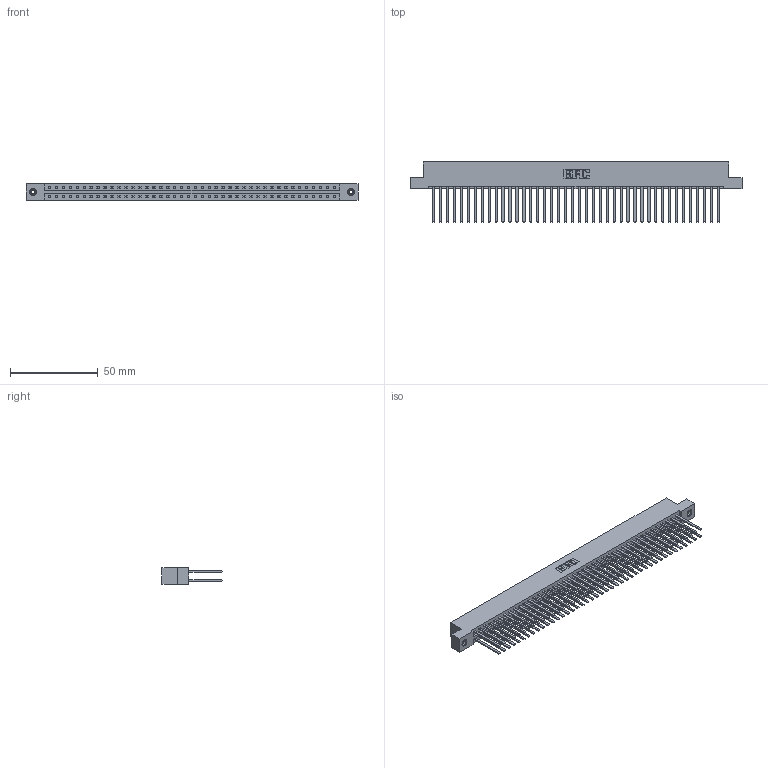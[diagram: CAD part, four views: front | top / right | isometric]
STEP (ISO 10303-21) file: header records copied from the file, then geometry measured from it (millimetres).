
FILE_DESCRIPTION (( 'STEP AP203' ), '1' );
FILE_NAME ('387-084-544-208.STEP', '2018-09-23T22:19:50', ( '' ), ( '' ), 'SwSTEP 2.0', 'SolidWorks 2016', '' );
FILE_SCHEMA (( 'CONFIG_CONTROL_DESIGN' ));
Length unit declared in the file: inch
Products named in the file (4): 337 Part_Flush Mounting Lugs - 0.156 Dia-TI; 345-292-001_345-293-144; 345-250-001_345-250-003-102; 387-084-544-208
Assembly tree (87 placements, depth 2):
  387-084-544-208
    337 Part_Flush Mounting Lugs - 0.156 Dia-TI
    345-292-001_345-293-144  x84
    345-250-001_345-250-003-102  x2
Bounding box: 189.43 x 34.3 x 9.4 mm (x, y, z)
Volume: 21135 mm3; surface area: 27763.7 mm2
Topology: 87 solids, 87 shells, 4206 faces, 12459 edges, 8186 vertices
Faces by surface type: plane 2958, cylinder 1232, cone 12, torus 4
Entity records: 33566 total; most frequent: CARTESIAN_POINT 5633, ORIENTED_EDGE 5562, DIRECTION 4819, EDGE_CURVE 2781, VECTOR 2637, LINE 2637, VERTEX_POINT 1848, AXIS2_PLACEMENT_3D 1091
